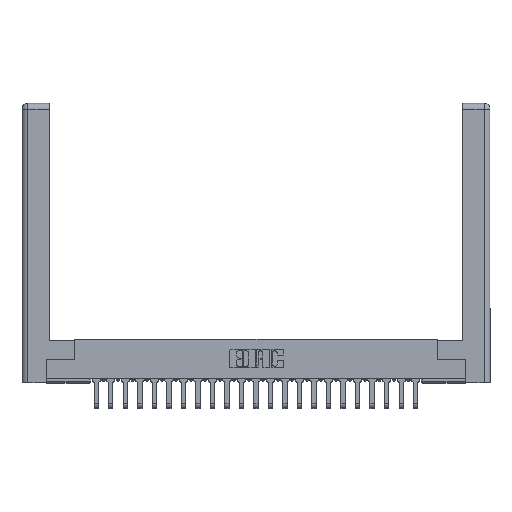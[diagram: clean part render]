
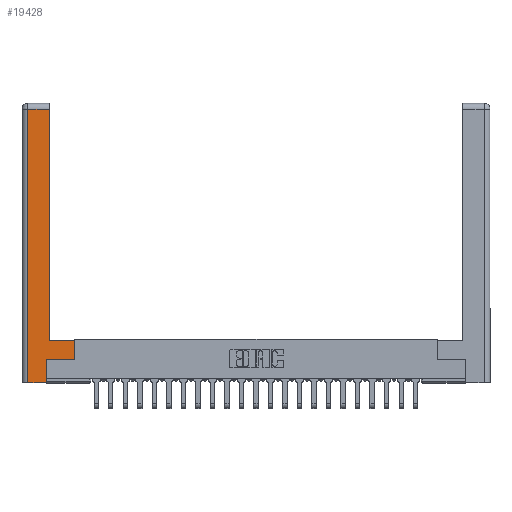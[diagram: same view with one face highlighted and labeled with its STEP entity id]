
A CAD part, top view. The second image highlights one B-rep face of the part: STEP entity #19428.
In plain terms, the highlighted planar face has unit normal (0, 0, 1).
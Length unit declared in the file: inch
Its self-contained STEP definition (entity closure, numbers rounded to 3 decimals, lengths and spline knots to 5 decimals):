
#68 = CARTESIAN_POINT ( 'NONE',  ( 0.265, 0.245, 0. ) ) ;
#439 = CARTESIAN_POINT ( 'NONE',  ( 0.295, 2.94, 0. ) ) ;
#748 = CARTESIAN_POINT ( 'NONE',  ( 0.0615, 0., 0. ) ) ;
#1758 = ORIENTED_EDGE ( 'NONE', *, *, #3377, .T. ) ;
#1985 = CARTESIAN_POINT ( 'NONE',  ( 0.265, 0.245, 0. ) ) ;
#2275 = DIRECTION ( 'NONE',  ( -1., 0., 0. ) ) ;
#2332 = EDGE_CURVE ( 'NONE', #4839, #15036, #15096, .T. ) ;
#2821 = ORIENTED_EDGE ( 'NONE', *, *, #10832, .T. ) ;
#3377 = EDGE_CURVE ( 'NONE', #13883, #6054, #14173, .T. ) ;
#3545 = CARTESIAN_POINT ( 'NONE',  ( 0.0615, 0., 0. ) ) ;
#3797 = ORIENTED_EDGE ( 'NONE', *, *, #6028, .T. ) ;
#4259 = ORIENTED_EDGE ( 'NONE', *, *, #2332, .T. ) ;
#4287 = LINE ( 'NONE', #13904, #15706 ) ;
#4321 = CARTESIAN_POINT ( 'NONE',  ( 0.565, 0.45, 0. ) ) ;
#4839 = VERTEX_POINT ( 'NONE', #21044 ) ;
#4869 = ORIENTED_EDGE ( 'NONE', *, *, #22142, .T. ) ;
#6028 = EDGE_CURVE ( 'NONE', #12320, #6084, #4287, .T. ) ;
#6054 = VERTEX_POINT ( 'NONE', #11918 ) ;
#6084 = VERTEX_POINT ( 'NONE', #4321 ) ;
#6124 = EDGE_CURVE ( 'NONE', #10096, #13883, #14832, .T. ) ;
#6697 = VECTOR ( 'NONE', #19827, 39.37008 ) ;
#6908 = CARTESIAN_POINT ( 'NONE',  ( 0.265, 0., 0. ) ) ;
#7016 = CARTESIAN_POINT ( 'NONE',  ( 0.565, 0.245, 0. ) ) ;
#7599 = LINE ( 'NONE', #6908, #9130 ) ;
#8856 = ORIENTED_EDGE ( 'NONE', *, *, #6124, .T. ) ;
#9130 = VECTOR ( 'NONE', #18458, 39.37008 ) ;
#10027 = VECTOR ( 'NONE', #11784, 39.37008 ) ;
#10083 = CARTESIAN_POINT ( 'NONE',  ( 0.295, 3., 0. ) ) ;
#10096 = VERTEX_POINT ( 'NONE', #23582 ) ;
#10832 = EDGE_CURVE ( 'NONE', #19401, #4839, #7599, .T. ) ;
#11742 = DIRECTION ( 'NONE',  ( 0., 0., -1. ) ) ;
#11743 = VECTOR ( 'NONE', #19646, 39.37008 ) ;
#11784 = DIRECTION ( 'NONE',  ( 0., 1., 0. ) ) ;
#11918 = CARTESIAN_POINT ( 'NONE',  ( 0.0615, 2.94, 0. ) ) ;
#12035 = DIRECTION ( 'NONE',  ( 0., -1., 0. ) ) ;
#12320 = VERTEX_POINT ( 'NONE', #22822 ) ;
#12587 = EDGE_CURVE ( 'NONE', #6084, #10096, #19481, .T. ) ;
#13383 = PLANE ( 'NONE',  #15732 ) ;
#13658 = DIRECTION ( 'NONE',  ( 0., 1., 0. ) ) ;
#13883 = VERTEX_POINT ( 'NONE', #439 ) ;
#13904 = CARTESIAN_POINT ( 'NONE',  ( 0.565, 0.45, 0. ) ) ;
#13959 = CARTESIAN_POINT ( 'NONE',  ( 0.295, 0.45, 0. ) ) ;
#14173 = LINE ( 'NONE', #20364, #20729 ) ;
#14209 = EDGE_LOOP ( 'NONE', ( #8856, #1758, #4869, #2821, #4259, #19113, #3797, #17255 ) ) ;
#14493 = FACE_OUTER_BOUND ( 'NONE', #14209, .T. ) ;
#14832 = LINE ( 'NONE', #10083, #6697 ) ;
#14867 = DIRECTION ( 'NONE',  ( -1., 0., 0. ) ) ;
#15036 = VERTEX_POINT ( 'NONE', #1985 ) ;
#15096 = LINE ( 'NONE', #68, #10027 ) ;
#15706 = VECTOR ( 'NONE', #13658, 39.37008 ) ;
#15732 = AXIS2_PLACEMENT_3D ( 'NONE', #17717, #11742, #2275 ) ;
#17255 = ORIENTED_EDGE ( 'NONE', *, *, #12587, .T. ) ;
#17717 = CARTESIAN_POINT ( 'NONE',  ( 0., 0., 0. ) ) ;
#17739 = EDGE_CURVE ( 'NONE', #15036, #12320, #19930, .T. ) ;
#17974 = VECTOR ( 'NONE', #12035, 39.37008 ) ;
#18458 = DIRECTION ( 'NONE',  ( 1., 0., 0. ) ) ;
#19113 = ORIENTED_EDGE ( 'NONE', *, *, #17739, .T. ) ;
#19401 = VERTEX_POINT ( 'NONE', #3545 ) ;
#19428 = ADVANCED_FACE ( 'NONE', ( #14493 ), #13383, .F. ) ;
#19481 = LINE ( 'NONE', #13959, #11743 ) ;
#19646 = DIRECTION ( 'NONE',  ( -1., 0., 0. ) ) ;
#19827 = DIRECTION ( 'NONE',  ( 0., 1., 0. ) ) ;
#19930 = LINE ( 'NONE', #7016, #24094 ) ;
#20364 = CARTESIAN_POINT ( 'NONE',  ( 0.0615, 2.94, 0. ) ) ;
#20729 = VECTOR ( 'NONE', #14867, 39.37008 ) ;
#21044 = CARTESIAN_POINT ( 'NONE',  ( 0.265, 0., 0. ) ) ;
#22142 = EDGE_CURVE ( 'NONE', #6054, #19401, #23059, .T. ) ;
#22232 = DIRECTION ( 'NONE',  ( 1., 0., 0. ) ) ;
#22822 = CARTESIAN_POINT ( 'NONE',  ( 0.565, 0.245, 0. ) ) ;
#23059 = LINE ( 'NONE', #748, #17974 ) ;
#23582 = CARTESIAN_POINT ( 'NONE',  ( 0.295, 0.45, 0. ) ) ;
#24094 = VECTOR ( 'NONE', #22232, 39.37008 ) ;
